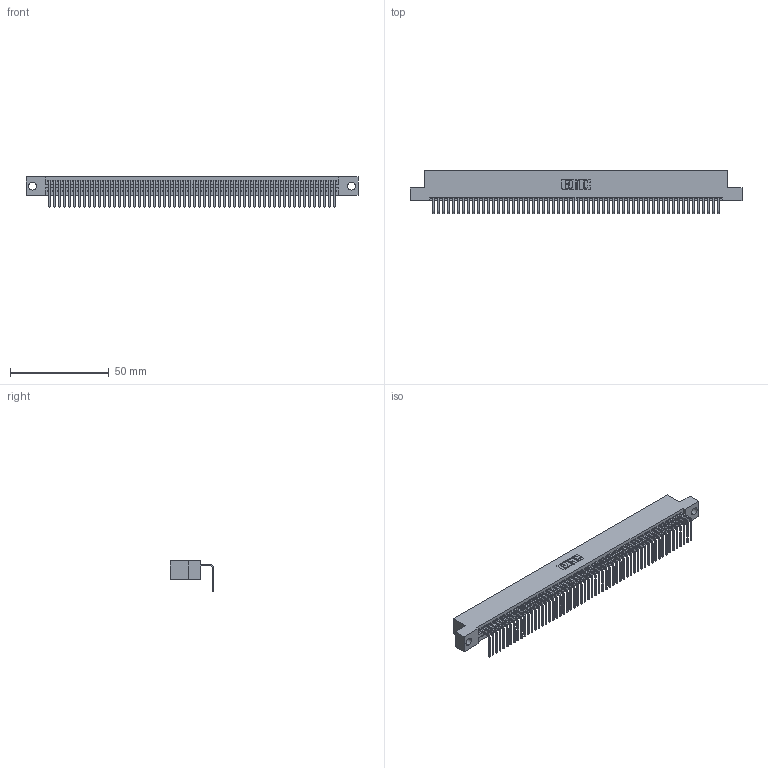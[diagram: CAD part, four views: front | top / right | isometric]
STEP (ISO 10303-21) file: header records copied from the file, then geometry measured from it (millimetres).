
FILE_DESCRIPTION (( 'STEP AP203' ), '1' );
FILE_NAME ('345-058-558-104.STEP', '2021-06-10T14:49:17', ( '' ), ( '' ), 'SwSTEP 2.0', 'SolidWorks 2020', '' );
FILE_SCHEMA (( 'CONFIG_CONTROL_DESIGN' ));
Length unit declared in the file: inch
Products named in the file (3): 345-292-001_558 Tail - 2; 345 Part_Flush Mounting Lugs - 0.156 Dia-TI; 345-058-558-104
Assembly tree (59 placements, depth 2):
  345-058-558-104
    345 Part_Flush Mounting Lugs - 0.156 Dia-TI
    345-292-001_558 Tail - 2  x58
Bounding box: 168.53 x 21.83 x 15.37 mm (x, y, z)
Volume: 16225.4 mm3; surface area: 22757.6 mm2
Topology: 59 solids, 59 shells, 3620 faces, 10933 edges, 7210 vertices
Faces by surface type: plane 2530, cylinder 1090
Entity records: 42001 total; most frequent: CARTESIAN_POINT 7284, ORIENTED_EDGE 7274, DIRECTION 6337, EDGE_CURVE 3637, VECTOR 3273, LINE 3273, VERTEX_POINT 2422, AXIS2_PLACEMENT_3D 1532
